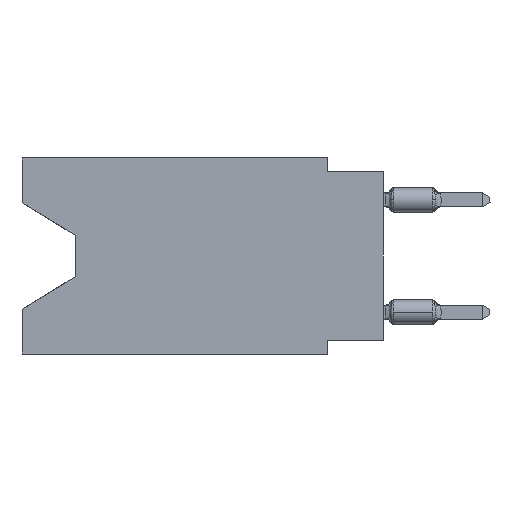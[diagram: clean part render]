
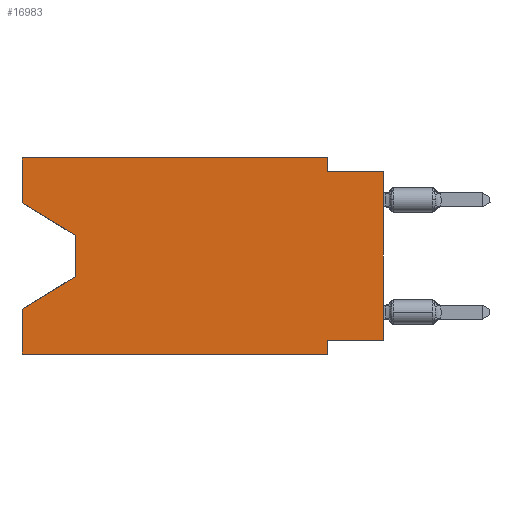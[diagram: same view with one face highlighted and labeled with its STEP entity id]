
A CAD part, left-side view. The second image highlights one B-rep face of the part: STEP entity #16983.
In plain terms, the highlighted planar face has unit normal (-1, 0, 0).
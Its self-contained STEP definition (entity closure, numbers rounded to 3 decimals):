
#444 = EDGE_CURVE ( 'NONE', #21922, #11202, #12579, .T. ) ;
#591 = EDGE_CURVE ( 'NONE', #2208, #15946, #23450, .T. ) ;
#719 = EDGE_CURVE ( 'NONE', #25297, #22448, #18001, .T. ) ;
#919 = CARTESIAN_POINT ( 'NONE',  ( 0., 0., -0.635 ) ) ;
#935 = FACE_OUTER_BOUND ( 'NONE', #4297, .T. ) ;
#954 = CARTESIAN_POINT ( 'NONE',  ( 0., 0., -0.635 ) ) ;
#1695 = CARTESIAN_POINT ( 'NONE',  ( 0., 2.54, -8.89 ) ) ;
#2208 = VERTEX_POINT ( 'NONE', #16906 ) ;
#2315 = EDGE_CURVE ( 'NONE', #8359, #15807, #25284, .T. ) ;
#2512 = ORIENTED_EDGE ( 'NONE', *, *, #20073, .F. ) ;
#2777 = DIRECTION ( 'NONE',  ( 0., 1., 0. ) ) ;
#2971 = VERTEX_POINT ( 'NONE', #26196 ) ;
#3139 = VECTOR ( 'NONE', #7840, 1000. ) ;
#3207 = CARTESIAN_POINT ( 'NONE',  ( 0., 16.383, 0. ) ) ;
#3240 = ORIENTED_EDGE ( 'NONE', *, *, #11448, .F. ) ;
#3551 = VECTOR ( 'NONE', #26128, 1000. ) ;
#3628 = VECTOR ( 'NONE', #19609, 1000. ) ;
#3773 = ORIENTED_EDGE ( 'NONE', *, *, #591, .F. ) ;
#3871 = EDGE_CURVE ( 'NONE', #22787, #2971, #20230, .T. ) ;
#3966 = ORIENTED_EDGE ( 'NONE', *, *, #2315, .F. ) ;
#4297 = EDGE_LOOP ( 'NONE', ( #21677, #16472, #10964, #6485, #16278, #3966, #16826, #11458, #3240, #3773, #2512, #9846 ) ) ;
#5026 = DIRECTION ( 'NONE',  ( 0., 0., 1. ) ) ;
#5578 = CARTESIAN_POINT ( 'NONE',  ( 0., 16.383, -2.038 ) ) ;
#6485 = ORIENTED_EDGE ( 'NONE', *, *, #719, .F. ) ;
#7668 = VECTOR ( 'NONE', #26073, 1000. ) ;
#7840 = DIRECTION ( 'NONE',  ( 0., -0.855, -0.519 ) ) ;
#8359 = VERTEX_POINT ( 'NONE', #15130 ) ;
#8402 = CARTESIAN_POINT ( 'NONE',  ( 0., 0., -8.255 ) ) ;
#8432 = EDGE_CURVE ( 'NONE', #21922, #22787, #15664, .T. ) ;
#9183 = VERTEX_POINT ( 'NONE', #954 ) ;
#9188 = DIRECTION ( 'NONE',  ( 0., 0., -1. ) ) ;
#9846 = ORIENTED_EDGE ( 'NONE', *, *, #444, .F. ) ;
#10964 = ORIENTED_EDGE ( 'NONE', *, *, #11036, .T. ) ;
#11036 = EDGE_CURVE ( 'NONE', #2971, #22448, #19358, .T. ) ;
#11185 = VECTOR ( 'NONE', #20687, 1000. ) ;
#11202 = VERTEX_POINT ( 'NONE', #16367 ) ;
#11252 = CARTESIAN_POINT ( 'NONE',  ( 0., 13.97, -5.385 ) ) ;
#11448 = EDGE_CURVE ( 'NONE', #15946, #9183, #21659, .T. ) ;
#11458 = ORIENTED_EDGE ( 'NONE', *, *, #19943, .T. ) ;
#11629 = VECTOR ( 'NONE', #13457, 1000. ) ;
#11730 = VECTOR ( 'NONE', #5026, 1000. ) ;
#12574 = VECTOR ( 'NONE', #22435, 1000. ) ;
#12579 = LINE ( 'NONE', #16550, #11185 ) ;
#12822 = CARTESIAN_POINT ( 'NONE',  ( 0., 16.383, -8.89 ) ) ;
#13019 = DIRECTION ( 'NONE',  ( 0., -1., 0. ) ) ;
#13181 = CARTESIAN_POINT ( 'NONE',  ( 0., 2.54, -8.89 ) ) ;
#13434 = PLANE ( 'NONE',  #18206 ) ;
#13457 = DIRECTION ( 'NONE',  ( 0., 0., -1. ) ) ;
#13563 = VERTEX_POINT ( 'NONE', #8402 ) ;
#13737 = VECTOR ( 'NONE', #20938, 1000. ) ;
#14332 = LINE ( 'NONE', #23891, #12574 ) ;
#14459 = CARTESIAN_POINT ( 'NONE',  ( 0., 16.383, -6.852 ) ) ;
#15130 = CARTESIAN_POINT ( 'NONE',  ( 0., 2.54, -8.255 ) ) ;
#15664 = LINE ( 'NONE', #5578, #3139 ) ;
#15807 = VERTEX_POINT ( 'NONE', #1695 ) ;
#15946 = VERTEX_POINT ( 'NONE', #22038 ) ;
#16278 = ORIENTED_EDGE ( 'NONE', *, *, #19594, .T. ) ;
#16367 = CARTESIAN_POINT ( 'NONE',  ( 0., 16.383, 0. ) ) ;
#16472 = ORIENTED_EDGE ( 'NONE', *, *, #3871, .T. ) ;
#16550 = CARTESIAN_POINT ( 'NONE',  ( 0., 16.383, 0. ) ) ;
#16826 = ORIENTED_EDGE ( 'NONE', *, *, #21005, .F. ) ;
#16906 = CARTESIAN_POINT ( 'NONE',  ( 0., 2.54, 0. ) ) ;
#16983 = ADVANCED_FACE ( 'NONE', ( #935 ), #13434, .F. ) ;
#17139 = DIRECTION ( 'NONE',  ( 1., 0., 0. ) ) ;
#17438 = CARTESIAN_POINT ( 'NONE',  ( 0., 16.383, -2.038 ) ) ;
#17630 = VECTOR ( 'NONE', #20466, 1000. ) ;
#18001 = LINE ( 'NONE', #19870, #3551 ) ;
#18206 = AXIS2_PLACEMENT_3D ( 'NONE', #3207, #17139, #9188 ) ;
#18948 = CARTESIAN_POINT ( 'NONE',  ( 0., 2.54, 0. ) ) ;
#19273 = VECTOR ( 'NONE', #2777, 1000. ) ;
#19358 = LINE ( 'NONE', #11252, #3628 ) ;
#19594 = EDGE_CURVE ( 'NONE', #25297, #15807, #26197, .T. ) ;
#19609 = DIRECTION ( 'NONE',  ( 0., 0.855, -0.519 ) ) ;
#19823 = CARTESIAN_POINT ( 'NONE',  ( 0., 13.97, -3.505 ) ) ;
#19870 = CARTESIAN_POINT ( 'NONE',  ( 0., 16.383, 0. ) ) ;
#19943 = EDGE_CURVE ( 'NONE', #13563, #9183, #25892, .T. ) ;
#20073 = EDGE_CURVE ( 'NONE', #11202, #2208, #14332, .T. ) ;
#20230 = LINE ( 'NONE', #19823, #7668 ) ;
#20466 = DIRECTION ( 'NONE',  ( 0., -1., 0. ) ) ;
#20687 = DIRECTION ( 'NONE',  ( 0., 0., 1. ) ) ;
#20938 = DIRECTION ( 'NONE',  ( 0., 0., -1. ) ) ;
#20987 = LINE ( 'NONE', #23241, #19273 ) ;
#21005 = EDGE_CURVE ( 'NONE', #13563, #8359, #20987, .T. ) ;
#21177 = CARTESIAN_POINT ( 'NONE',  ( 0., 13.97, -3.505 ) ) ;
#21659 = LINE ( 'NONE', #919, #24827 ) ;
#21677 = ORIENTED_EDGE ( 'NONE', *, *, #8432, .T. ) ;
#21922 = VERTEX_POINT ( 'NONE', #17438 ) ;
#22038 = CARTESIAN_POINT ( 'NONE',  ( 0., 2.54, -0.635 ) ) ;
#22435 = DIRECTION ( 'NONE',  ( 0., -1., 0. ) ) ;
#22448 = VERTEX_POINT ( 'NONE', #14459 ) ;
#22787 = VERTEX_POINT ( 'NONE', #21177 ) ;
#23235 = CARTESIAN_POINT ( 'NONE',  ( 0., 0., 0. ) ) ;
#23241 = CARTESIAN_POINT ( 'NONE',  ( 0., 0., -8.255 ) ) ;
#23450 = LINE ( 'NONE', #18948, #13737 ) ;
#23891 = CARTESIAN_POINT ( 'NONE',  ( 0., 16.383, 0. ) ) ;
#24461 = CARTESIAN_POINT ( 'NONE',  ( 0., 16.383, -8.89 ) ) ;
#24827 = VECTOR ( 'NONE', #13019, 1000. ) ;
#25284 = LINE ( 'NONE', #13181, #11629 ) ;
#25297 = VERTEX_POINT ( 'NONE', #12822 ) ;
#25892 = LINE ( 'NONE', #23235, #11730 ) ;
#26073 = DIRECTION ( 'NONE',  ( 0., 0., -1. ) ) ;
#26128 = DIRECTION ( 'NONE',  ( 0., 0., 1. ) ) ;
#26196 = CARTESIAN_POINT ( 'NONE',  ( 0., 13.97, -5.385 ) ) ;
#26197 = LINE ( 'NONE', #24461, #17630 ) ;
